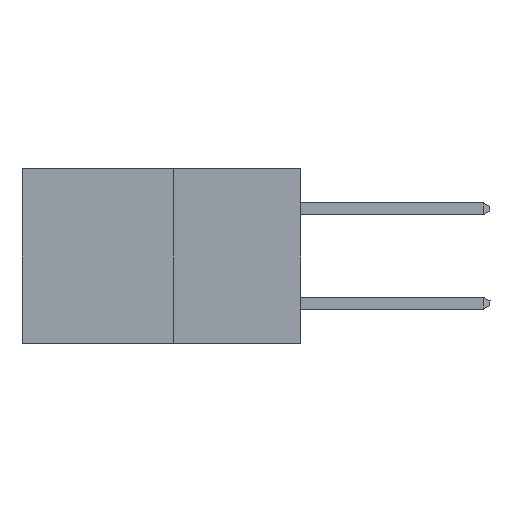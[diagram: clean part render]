
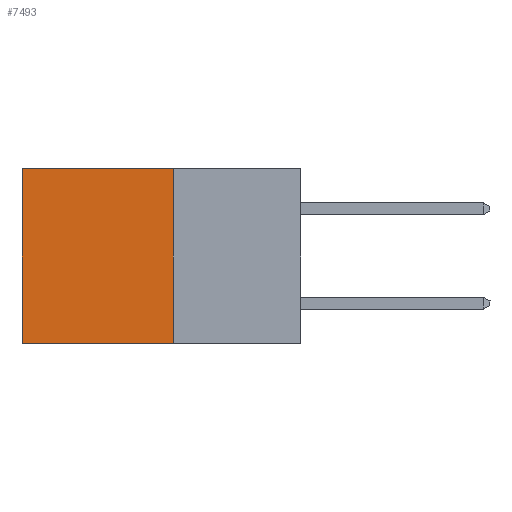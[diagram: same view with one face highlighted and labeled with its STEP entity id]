
A CAD part, left-side view. The second image highlights one B-rep face of the part: STEP entity #7493.
In plain terms, the highlighted planar face has unit normal (-1, 0, 0).
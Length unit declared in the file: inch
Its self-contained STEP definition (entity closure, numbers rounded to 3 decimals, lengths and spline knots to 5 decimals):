
#40 = EDGE_LOOP ( 'NONE', ( #5165, #17477, #18695, #16112 ) ) ;
#658 = VERTEX_POINT ( 'NONE', #29229 ) ;
#1457 = EDGE_CURVE ( 'NONE', #17847, #5672, #25409, .T. ) ;
#3460 = VECTOR ( 'NONE', #4478, 39.37008 ) ;
#4478 = DIRECTION ( 'NONE',  ( 0., 0., -1. ) ) ;
#5165 = ORIENTED_EDGE ( 'NONE', *, *, #18820, .T. ) ;
#5672 = VERTEX_POINT ( 'NONE', #19593 ) ;
#5743 = VECTOR ( 'NONE', #14602, 39.37008 ) ;
#7146 = DIRECTION ( 'NONE',  ( 0., 0., -1. ) ) ;
#7223 = DIRECTION ( 'NONE',  ( 1., 0., 0. ) ) ;
#7257 = PLANE ( 'NONE',  #11586 ) ;
#7493 = ADVANCED_FACE ( 'NONE', ( #8093 ), #7257, .F. ) ;
#7708 = CARTESIAN_POINT ( 'NONE',  ( 0.277, 0.27, -0.37 ) ) ;
#8093 = FACE_OUTER_BOUND ( 'NONE', #40, .T. ) ;
#8558 = CARTESIAN_POINT ( 'NONE',  ( 0.277, 0.27, 0. ) ) ;
#9413 = VECTOR ( 'NONE', #17045, 39.37008 ) ;
#9868 = VERTEX_POINT ( 'NONE', #12229 ) ;
#10323 = LINE ( 'NONE', #30013, #3460 ) ;
#11586 = AXIS2_PLACEMENT_3D ( 'NONE', #7708, #7223, #7146 ) ;
#12229 = CARTESIAN_POINT ( 'NONE',  ( 0.277, 0.59, -0.37 ) ) ;
#13438 = CARTESIAN_POINT ( 'NONE',  ( 0.277, 0.27, 0. ) ) ;
#14443 = DIRECTION ( 'NONE',  ( 0., 1., 0. ) ) ;
#14602 = DIRECTION ( 'NONE',  ( 0., 1., 0. ) ) ;
#16112 = ORIENTED_EDGE ( 'NONE', *, *, #1457, .T. ) ;
#16685 = EDGE_CURVE ( 'NONE', #658, #9868, #24368, .T. ) ;
#17045 = DIRECTION ( 'NONE',  ( 0., 0., -1. ) ) ;
#17477 = ORIENTED_EDGE ( 'NONE', *, *, #16685, .F. ) ;
#17484 = VECTOR ( 'NONE', #14443, 39.37008 ) ;
#17847 = VERTEX_POINT ( 'NONE', #8558 ) ;
#18695 = ORIENTED_EDGE ( 'NONE', *, *, #22648, .F. ) ;
#18820 = EDGE_CURVE ( 'NONE', #5672, #9868, #23020, .T. ) ;
#19593 = CARTESIAN_POINT ( 'NONE',  ( 0.277, 0.59, 0. ) ) ;
#22648 = EDGE_CURVE ( 'NONE', #17847, #658, #10323, .T. ) ;
#23020 = LINE ( 'NONE', #24740, #9413 ) ;
#24368 = LINE ( 'NONE', #27279, #17484 ) ;
#24740 = CARTESIAN_POINT ( 'NONE',  ( 0.277, 0.59, -0.37 ) ) ;
#25409 = LINE ( 'NONE', #13438, #5743 ) ;
#27279 = CARTESIAN_POINT ( 'NONE',  ( 0.277, 0.27, -0.37 ) ) ;
#29229 = CARTESIAN_POINT ( 'NONE',  ( 0.277, 0.27, -0.37 ) ) ;
#30013 = CARTESIAN_POINT ( 'NONE',  ( 0.277, 0.27, -0.37 ) ) ;
